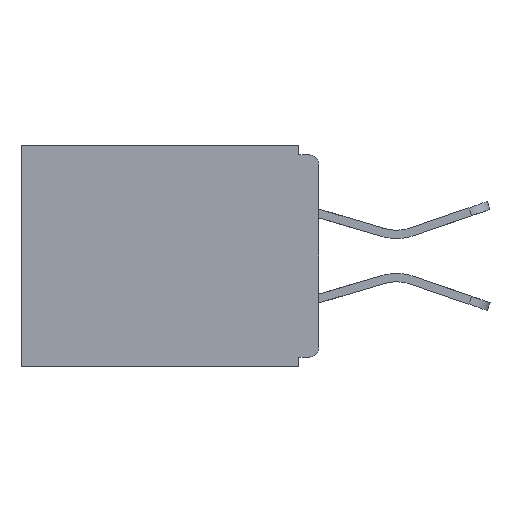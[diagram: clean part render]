
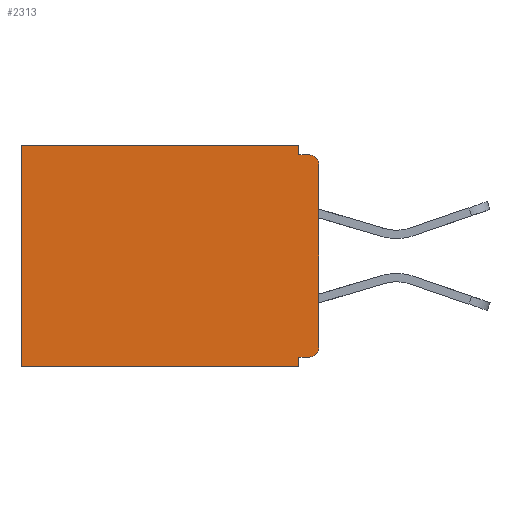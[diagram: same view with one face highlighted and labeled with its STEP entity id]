
A CAD part, left-side view. The second image highlights one B-rep face of the part: STEP entity #2313.
In plain terms, the highlighted planar face has unit normal (-1, 0, 0).
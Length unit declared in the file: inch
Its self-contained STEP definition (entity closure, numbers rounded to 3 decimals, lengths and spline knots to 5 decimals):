
#3 = AXIS2_PLACEMENT_3D ( 'NONE', #9722, #7818, #15863 ) ;
#228 = EDGE_CURVE ( 'NONE', #17021, #10133, #9375, .T. ) ;
#660 = CARTESIAN_POINT ( 'NONE',  ( 0.298, 0.015, -0.015 ) ) ;
#702 = VERTEX_POINT ( 'NONE', #13552 ) ;
#918 = VERTEX_POINT ( 'NONE', #10260 ) ;
#1226 = PLANE ( 'NONE',  #17537 ) ;
#1252 = EDGE_CURVE ( 'NONE', #20327, #14212, #1307, .T. ) ;
#1307 = LINE ( 'NONE', #2048, #17084 ) ;
#1361 = DIRECTION ( 'NONE',  ( 0., 0., -1. ) ) ;
#1373 = VECTOR ( 'NONE', #2392, 39.37008 ) ;
#1470 = CARTESIAN_POINT ( 'NONE',  ( 0.298, 0., 0. ) ) ;
#1961 = CARTESIAN_POINT ( 'NONE',  ( 0.298, 0., -0.343 ) ) ;
#2048 = CARTESIAN_POINT ( 'NONE',  ( 0.298, 0., -0.015 ) ) ;
#2058 = EDGE_CURVE ( 'NONE', #918, #21808, #19520, .T. ) ;
#2069 = ORIENTED_EDGE ( 'NONE', *, *, #1252, .F. ) ;
#2156 = LINE ( 'NONE', #10924, #6207 ) ;
#2313 = ADVANCED_FACE ( 'NONE', ( #23850 ), #1226, .F. ) ;
#2392 = DIRECTION ( 'NONE',  ( 0., 0., -1. ) ) ;
#2548 = ORIENTED_EDGE ( 'NONE', *, *, #10039, .T. ) ;
#2676 = DIRECTION ( 'NONE',  ( 0., 0., -1. ) ) ;
#4086 = ORIENTED_EDGE ( 'NONE', *, *, #19151, .F. ) ;
#4253 = LINE ( 'NONE', #5224, #24672 ) ;
#5224 = CARTESIAN_POINT ( 'NONE',  ( 0.298, 0., -0.328 ) ) ;
#5609 = ORIENTED_EDGE ( 'NONE', *, *, #20740, .F. ) ;
#5648 = CARTESIAN_POINT ( 'NONE',  ( 0.298, 0., -0.03 ) ) ;
#5699 = VERTEX_POINT ( 'NONE', #13315 ) ;
#6207 = VECTOR ( 'NONE', #23424, 39.37008 ) ;
#6969 = VECTOR ( 'NONE', #1361, 39.37008 ) ;
#7122 = CARTESIAN_POINT ( 'NONE',  ( 0.298, 0.031, 0. ) ) ;
#7818 = DIRECTION ( 'NONE',  ( -1., 0., 0. ) ) ;
#8576 = DIRECTION ( 'NONE',  ( 0., 0., -1. ) ) ;
#9254 = DIRECTION ( 'NONE',  ( 0., 0., -1. ) ) ;
#9375 = LINE ( 'NONE', #24103, #19562 ) ;
#9722 = CARTESIAN_POINT ( 'NONE',  ( 0.298, 0.015, -0.313 ) ) ;
#10039 = EDGE_CURVE ( 'NONE', #702, #5699, #24773, .T. ) ;
#10133 = VERTEX_POINT ( 'NONE', #24329 ) ;
#10260 = CARTESIAN_POINT ( 'NONE',  ( 0.298, 0.46, 0. ) ) ;
#10396 = LINE ( 'NONE', #16373, #1373 ) ;
#10924 = CARTESIAN_POINT ( 'NONE',  ( 0.298, 0., 0. ) ) ;
#11474 = ORIENTED_EDGE ( 'NONE', *, *, #18922, .F. ) ;
#11632 = ORIENTED_EDGE ( 'NONE', *, *, #25578, .F. ) ;
#12246 = LINE ( 'NONE', #1961, #22105 ) ;
#12267 = LINE ( 'NONE', #15385, #6969 ) ;
#13315 = CARTESIAN_POINT ( 'NONE',  ( 0.298, 0., -0.313 ) ) ;
#13552 = CARTESIAN_POINT ( 'NONE',  ( 0.298, 0.015, -0.328 ) ) ;
#13686 = VECTOR ( 'NONE', #8576, 39.37008 ) ;
#14107 = DIRECTION ( 'NONE',  ( 0., 0., -1. ) ) ;
#14212 = VERTEX_POINT ( 'NONE', #660 ) ;
#14598 = EDGE_CURVE ( 'NONE', #20044, #14212, #14918, .T. ) ;
#14918 = CIRCLE ( 'NONE', #23864, 0.015 ) ;
#15066 = DIRECTION ( 'NONE',  ( 1., 0., 0. ) ) ;
#15180 = ORIENTED_EDGE ( 'NONE', *, *, #16988, .T. ) ;
#15385 = CARTESIAN_POINT ( 'NONE',  ( 0.298, 0., 0. ) ) ;
#15716 = DIRECTION ( 'NONE',  ( 0., 1., 0. ) ) ;
#15863 = DIRECTION ( 'NONE',  ( 0., 0., -1. ) ) ;
#16373 = CARTESIAN_POINT ( 'NONE',  ( 0.298, 0.031, -0.343 ) ) ;
#16576 = CARTESIAN_POINT ( 'NONE',  ( 0.298, 0.015, -0.03 ) ) ;
#16651 = DIRECTION ( 'NONE',  ( -1., 0., 0. ) ) ;
#16879 = CARTESIAN_POINT ( 'NONE',  ( 0.298, 0.46, 0. ) ) ;
#16988 = EDGE_CURVE ( 'NONE', #17385, #918, #2156, .T. ) ;
#17021 = VERTEX_POINT ( 'NONE', #25444 ) ;
#17084 = VECTOR ( 'NONE', #25499, 39.37008 ) ;
#17385 = VERTEX_POINT ( 'NONE', #7122 ) ;
#17537 = AXIS2_PLACEMENT_3D ( 'NONE', #1470, #15066, #9254 ) ;
#18084 = ORIENTED_EDGE ( 'NONE', *, *, #14598, .T. ) ;
#18922 = EDGE_CURVE ( 'NONE', #20044, #5699, #12267, .T. ) ;
#19026 = DIRECTION ( 'NONE',  ( 0., 1., 0. ) ) ;
#19151 = EDGE_CURVE ( 'NONE', #17385, #20327, #10396, .T. ) ;
#19492 = CARTESIAN_POINT ( 'NONE',  ( 0.298, 0.46, -0.343 ) ) ;
#19520 = LINE ( 'NONE', #16879, #13686 ) ;
#19562 = VECTOR ( 'NONE', #14107, 39.37008 ) ;
#19780 = ORIENTED_EDGE ( 'NONE', *, *, #228, .F. ) ;
#20044 = VERTEX_POINT ( 'NONE', #5648 ) ;
#20327 = VERTEX_POINT ( 'NONE', #24477 ) ;
#20537 = EDGE_LOOP ( 'NONE', ( #18084, #2069, #4086, #15180, #23245, #5609, #19780, #11632, #2548, #11474 ) ) ;
#20740 = EDGE_CURVE ( 'NONE', #10133, #21808, #12246, .T. ) ;
#21808 = VERTEX_POINT ( 'NONE', #19492 ) ;
#22105 = VECTOR ( 'NONE', #15716, 39.37008 ) ;
#23245 = ORIENTED_EDGE ( 'NONE', *, *, #2058, .T. ) ;
#23424 = DIRECTION ( 'NONE',  ( 0., 1., 0. ) ) ;
#23850 = FACE_OUTER_BOUND ( 'NONE', #20537, .T. ) ;
#23864 = AXIS2_PLACEMENT_3D ( 'NONE', #16576, #16651, #2676 ) ;
#24103 = CARTESIAN_POINT ( 'NONE',  ( 0.298, 0.031, -0.343 ) ) ;
#24329 = CARTESIAN_POINT ( 'NONE',  ( 0.298, 0.031, -0.343 ) ) ;
#24477 = CARTESIAN_POINT ( 'NONE',  ( 0.298, 0.031, -0.015 ) ) ;
#24672 = VECTOR ( 'NONE', #19026, 39.37008 ) ;
#24773 = CIRCLE ( 'NONE', #3, 0.015 ) ;
#25444 = CARTESIAN_POINT ( 'NONE',  ( 0.298, 0.031, -0.328 ) ) ;
#25499 = DIRECTION ( 'NONE',  ( 0., -1., 0. ) ) ;
#25578 = EDGE_CURVE ( 'NONE', #702, #17021, #4253, .T. ) ;
